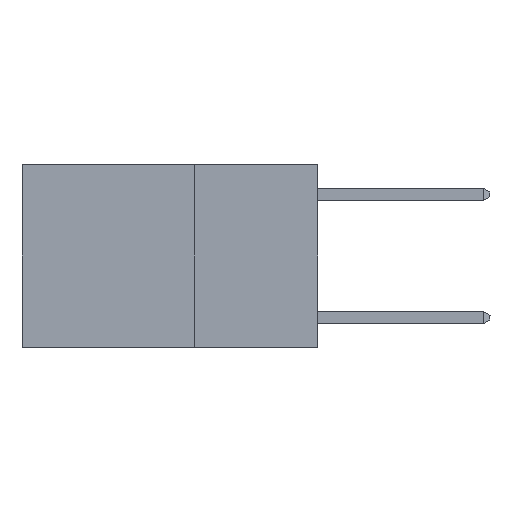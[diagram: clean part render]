
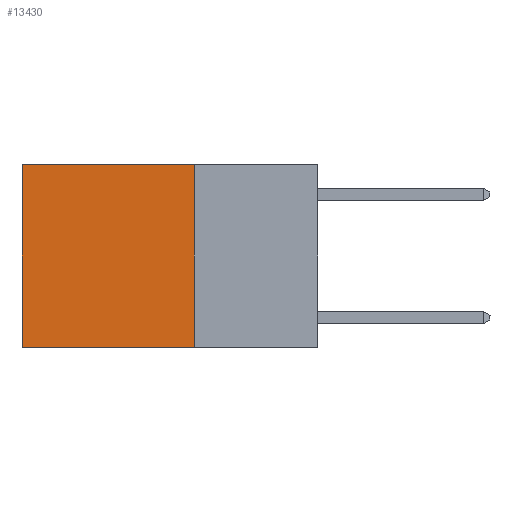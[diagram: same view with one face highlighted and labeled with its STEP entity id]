
A CAD part, left-side view. The second image highlights one B-rep face of the part: STEP entity #13430.
In plain terms, the highlighted planar face has unit normal (-1, 0, 0).
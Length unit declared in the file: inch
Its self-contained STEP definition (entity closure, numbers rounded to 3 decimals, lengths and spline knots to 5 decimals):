
#1170 = LINE ( 'NONE', #12018, #5654 ) ;
#1484 = VECTOR ( 'NONE', #14226, 39.37008 ) ;
#1647 = CARTESIAN_POINT ( 'NONE',  ( 0.2625, 0.25, 0. ) ) ;
#1947 = CARTESIAN_POINT ( 'NONE',  ( 0.2625, 0.25, 0. ) ) ;
#2169 = EDGE_CURVE ( 'NONE', #16778, #5874, #2291, .T. ) ;
#2291 = LINE ( 'NONE', #13074, #13552 ) ;
#3190 = DIRECTION ( 'NONE',  ( 0., 0., -1. ) ) ;
#3419 = PLANE ( 'NONE',  #6916 ) ;
#3491 = DIRECTION ( 'NONE',  ( 0., 0., -1. ) ) ;
#4429 = ORIENTED_EDGE ( 'NONE', *, *, #8079, .F. ) ;
#5392 = ORIENTED_EDGE ( 'NONE', *, *, #12917, .F. ) ;
#5654 = VECTOR ( 'NONE', #3190, 39.37008 ) ;
#5726 = CARTESIAN_POINT ( 'NONE',  ( 0.2625, 0.25, -0.37 ) ) ;
#5874 = VERTEX_POINT ( 'NONE', #8798 ) ;
#6916 = AXIS2_PLACEMENT_3D ( 'NONE', #1947, #12305, #3491 ) ;
#7922 = FACE_OUTER_BOUND ( 'NONE', #17216, .T. ) ;
#7963 = ORIENTED_EDGE ( 'NONE', *, *, #15702, .T. ) ;
#8079 = EDGE_CURVE ( 'NONE', #17614, #17550, #1170, .T. ) ;
#8798 = CARTESIAN_POINT ( 'NONE',  ( 0.2625, 0.6, -0.37 ) ) ;
#11337 = DIRECTION ( 'NONE',  ( 0., 1., 0. ) ) ;
#11659 = DIRECTION ( 'NONE',  ( 0., 0., -1. ) ) ;
#11906 = LINE ( 'NONE', #18366, #1484 ) ;
#12018 = CARTESIAN_POINT ( 'NONE',  ( 0.2625, 0.25, 0. ) ) ;
#12305 = DIRECTION ( 'NONE',  ( 1., 0., 0. ) ) ;
#12917 = EDGE_CURVE ( 'NONE', #17550, #5874, #13438, .T. ) ;
#13074 = CARTESIAN_POINT ( 'NONE',  ( 0.2625, 0.6, 0. ) ) ;
#13430 = ADVANCED_FACE ( 'NONE', ( #7922 ), #3419, .F. ) ;
#13438 = LINE ( 'NONE', #15605, #16749 ) ;
#13552 = VECTOR ( 'NONE', #11659, 39.37008 ) ;
#14226 = DIRECTION ( 'NONE',  ( 0., 1., 0. ) ) ;
#15328 = ORIENTED_EDGE ( 'NONE', *, *, #2169, .T. ) ;
#15605 = CARTESIAN_POINT ( 'NONE',  ( 0.2625, 0.25, -0.37 ) ) ;
#15702 = EDGE_CURVE ( 'NONE', #17614, #16778, #11906, .T. ) ;
#15751 = CARTESIAN_POINT ( 'NONE',  ( 0.2625, 0.6, 0. ) ) ;
#16749 = VECTOR ( 'NONE', #11337, 39.37008 ) ;
#16778 = VERTEX_POINT ( 'NONE', #15751 ) ;
#17216 = EDGE_LOOP ( 'NONE', ( #15328, #5392, #4429, #7963 ) ) ;
#17550 = VERTEX_POINT ( 'NONE', #5726 ) ;
#17614 = VERTEX_POINT ( 'NONE', #1647 ) ;
#18366 = CARTESIAN_POINT ( 'NONE',  ( 0.2625, 0.25, 0. ) ) ;
